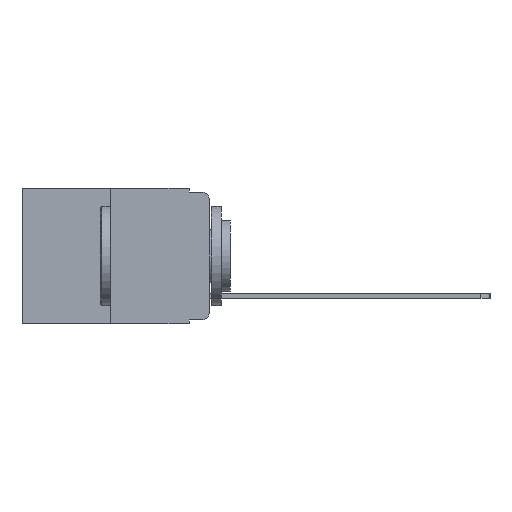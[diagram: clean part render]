
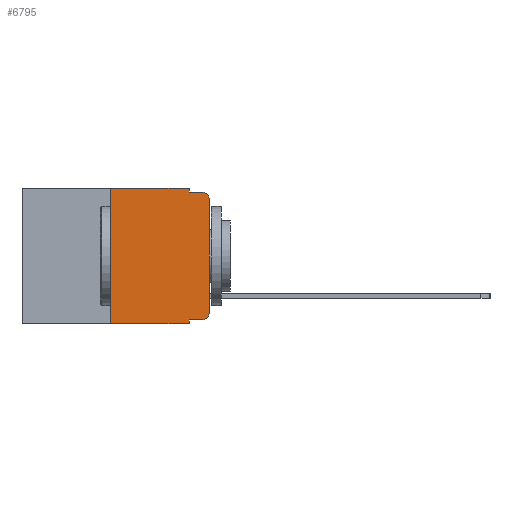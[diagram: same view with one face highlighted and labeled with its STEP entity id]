
A CAD part, left-side view. The second image highlights one B-rep face of the part: STEP entity #6795.
In plain terms, the highlighted planar face has unit normal (-1, 0, 0).
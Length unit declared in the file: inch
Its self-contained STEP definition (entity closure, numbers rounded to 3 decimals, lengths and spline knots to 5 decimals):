
#66 = VERTEX_POINT ( 'NONE', #12390 ) ;
#69 = DIRECTION ( 'NONE',  ( 0., 0., 1. ) ) ;
#137 = VERTEX_POINT ( 'NONE', #4013 ) ;
#811 = EDGE_CURVE ( 'NONE', #13903, #11483, #21008, .T. ) ;
#1699 = CARTESIAN_POINT ( 'NONE',  ( 0., 0.051, 0. ) ) ;
#2108 = EDGE_CURVE ( 'NONE', #137, #19426, #12083, .T. ) ;
#2191 = VECTOR ( 'NONE', #21853, 39.37008 ) ;
#2274 = ORIENTED_EDGE ( 'NONE', *, *, #20526, .T. ) ;
#2326 = VECTOR ( 'NONE', #14329, 39.37008 ) ;
#2557 = VECTOR ( 'NONE', #20644, 39.37008 ) ;
#2569 = CARTESIAN_POINT ( 'NONE',  ( 0., 0.25, 0. ) ) ;
#2995 = VECTOR ( 'NONE', #69, 39.37008 ) ;
#3034 = VERTEX_POINT ( 'NONE', #11702 ) ;
#3333 = DIRECTION ( 'NONE',  ( -1., 0., 0. ) ) ;
#3380 = EDGE_CURVE ( 'NONE', #66, #19722, #12276, .T. ) ;
#3473 = ORIENTED_EDGE ( 'NONE', *, *, #811, .F. ) ;
#3809 = VERTEX_POINT ( 'NONE', #21405 ) ;
#4013 = CARTESIAN_POINT ( 'NONE',  ( 0., 0.25, -0.343 ) ) ;
#4042 = ORIENTED_EDGE ( 'NONE', *, *, #8289, .T. ) ;
#5061 = EDGE_LOOP ( 'NONE', ( #4042, #5152, #5328, #10103, #10747, #5810, #2274, #3473, #12336, #22095 ) ) ;
#5152 = ORIENTED_EDGE ( 'NONE', *, *, #7073, .T. ) ;
#5256 = EDGE_CURVE ( 'NONE', #19426, #66, #9150, .T. ) ;
#5328 = ORIENTED_EDGE ( 'NONE', *, *, #5842, .F. ) ;
#5476 = LINE ( 'NONE', #9842, #14350 ) ;
#5505 = CARTESIAN_POINT ( 'NONE',  ( 0., 0.051, -0.01 ) ) ;
#5810 = ORIENTED_EDGE ( 'NONE', *, *, #2108, .F. ) ;
#5842 = EDGE_CURVE ( 'NONE', #19722, #18188, #7689, .T. ) ;
#6398 = CARTESIAN_POINT ( 'NONE',  ( 0., 0.473, 0. ) ) ;
#6795 = ADVANCED_FACE ( 'NONE', ( #20609 ), #7990, .F. ) ;
#7073 = EDGE_CURVE ( 'NONE', #11369, #18188, #20328, .T. ) ;
#7534 = VECTOR ( 'NONE', #19370, 39.37008 ) ;
#7689 = LINE ( 'NONE', #8127, #2191 ) ;
#7748 = CARTESIAN_POINT ( 'NONE',  ( 0., 0.02, -0.313 ) ) ;
#7990 = PLANE ( 'NONE',  #20102 ) ;
#8127 = CARTESIAN_POINT ( 'NONE',  ( 0., 0.051, -0.01 ) ) ;
#8164 = VECTOR ( 'NONE', #8561, 39.37008 ) ;
#8289 = EDGE_CURVE ( 'NONE', #3809, #11369, #17343, .T. ) ;
#8561 = DIRECTION ( 'NONE',  ( 0., 0., 1. ) ) ;
#9150 = LINE ( 'NONE', #6398, #20105 ) ;
#9565 = DIRECTION ( 'NONE',  ( 0., 0., -1. ) ) ;
#9822 = DIRECTION ( 'NONE',  ( 1., 0., 0. ) ) ;
#9842 = CARTESIAN_POINT ( 'NONE',  ( 0., 0.473, -0.343 ) ) ;
#10103 = ORIENTED_EDGE ( 'NONE', *, *, #3380, .F. ) ;
#10747 = ORIENTED_EDGE ( 'NONE', *, *, #5256, .F. ) ;
#11118 = CARTESIAN_POINT ( 'NONE',  ( 0., 0.25, 0. ) ) ;
#11369 = VERTEX_POINT ( 'NONE', #22732 ) ;
#11483 = VERTEX_POINT ( 'NONE', #12898 ) ;
#11613 = DIRECTION ( 'NONE',  ( 0., -1., 0. ) ) ;
#11702 = CARTESIAN_POINT ( 'NONE',  ( 0., 0.02, -0.333 ) ) ;
#11756 = AXIS2_PLACEMENT_3D ( 'NONE', #14060, #3333, #15740 ) ;
#12083 = LINE ( 'NONE', #11118, #2995 ) ;
#12230 = LINE ( 'NONE', #18935, #2557 ) ;
#12276 = LINE ( 'NONE', #1699, #7534 ) ;
#12303 = CARTESIAN_POINT ( 'NONE',  ( 0., 0.02, -0.01 ) ) ;
#12336 = ORIENTED_EDGE ( 'NONE', *, *, #20223, .T. ) ;
#12390 = CARTESIAN_POINT ( 'NONE',  ( 0., 0.051, 0. ) ) ;
#12464 = CARTESIAN_POINT ( 'NONE',  ( 0., 0.051, -0.333 ) ) ;
#12898 = CARTESIAN_POINT ( 'NONE',  ( 0., 0.051, -0.343 ) ) ;
#13903 = VERTEX_POINT ( 'NONE', #12464 ) ;
#14060 = CARTESIAN_POINT ( 'NONE',  ( 0., 0.02, -0.03 ) ) ;
#14329 = DIRECTION ( 'NONE',  ( 0., 0., -1. ) ) ;
#14350 = VECTOR ( 'NONE', #11613, 39.37008 ) ;
#14782 = AXIS2_PLACEMENT_3D ( 'NONE', #7748, #19772, #9565 ) ;
#15163 = DIRECTION ( 'NONE',  ( 0., -1., 0. ) ) ;
#15740 = DIRECTION ( 'NONE',  ( 0., 0., -1. ) ) ;
#17091 = CIRCLE ( 'NONE', #14782, 0.02 ) ;
#17343 = LINE ( 'NONE', #20483, #8164 ) ;
#18188 = VERTEX_POINT ( 'NONE', #12303 ) ;
#18322 = CARTESIAN_POINT ( 'NONE',  ( 0., 0.473, 0. ) ) ;
#18935 = CARTESIAN_POINT ( 'NONE',  ( 0., 0.051, -0.333 ) ) ;
#19097 = EDGE_CURVE ( 'NONE', #3034, #3809, #17091, .T. ) ;
#19370 = DIRECTION ( 'NONE',  ( 0., 0., -1. ) ) ;
#19426 = VERTEX_POINT ( 'NONE', #2569 ) ;
#19722 = VERTEX_POINT ( 'NONE', #5505 ) ;
#19772 = DIRECTION ( 'NONE',  ( -1., 0., 0. ) ) ;
#20102 = AXIS2_PLACEMENT_3D ( 'NONE', #18322, #9822, #21721 ) ;
#20105 = VECTOR ( 'NONE', #15163, 39.37008 ) ;
#20223 = EDGE_CURVE ( 'NONE', #13903, #3034, #12230, .T. ) ;
#20328 = CIRCLE ( 'NONE', #11756, 0.02 ) ;
#20483 = CARTESIAN_POINT ( 'NONE',  ( 0., 0., 0. ) ) ;
#20526 = EDGE_CURVE ( 'NONE', #137, #11483, #5476, .T. ) ;
#20609 = FACE_OUTER_BOUND ( 'NONE', #5061, .T. ) ;
#20644 = DIRECTION ( 'NONE',  ( 0., -1., 0. ) ) ;
#21008 = LINE ( 'NONE', #22726, #2326 ) ;
#21405 = CARTESIAN_POINT ( 'NONE',  ( 0., 0., -0.313 ) ) ;
#21721 = DIRECTION ( 'NONE',  ( 0., 0., -1. ) ) ;
#21853 = DIRECTION ( 'NONE',  ( 0., -1., 0. ) ) ;
#22095 = ORIENTED_EDGE ( 'NONE', *, *, #19097, .T. ) ;
#22726 = CARTESIAN_POINT ( 'NONE',  ( 0., 0.051, 0. ) ) ;
#22732 = CARTESIAN_POINT ( 'NONE',  ( 0., 0., -0.03 ) ) ;
